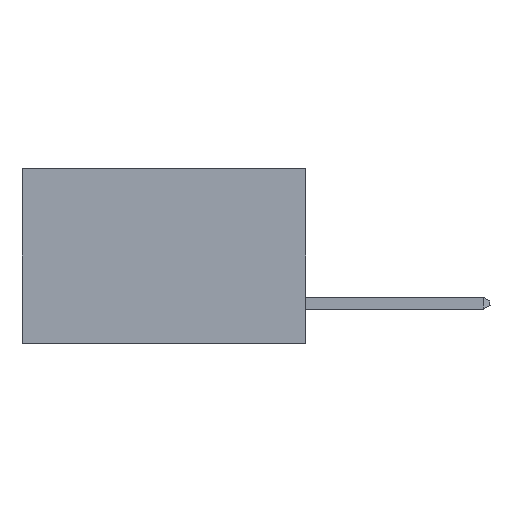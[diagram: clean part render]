
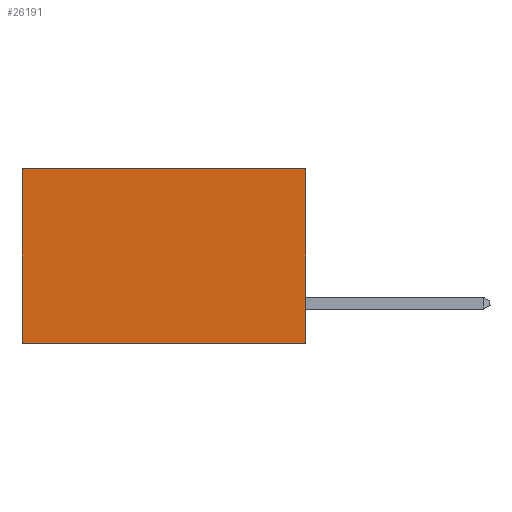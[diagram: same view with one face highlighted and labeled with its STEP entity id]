
A CAD part, left-side view. The second image highlights one B-rep face of the part: STEP entity #26191.
In plain terms, the highlighted planar face has unit normal (-1, 0, 0).
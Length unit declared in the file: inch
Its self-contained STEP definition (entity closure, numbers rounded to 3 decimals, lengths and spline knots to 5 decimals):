
#426 = CARTESIAN_POINT ( 'NONE',  ( 0.298, 0.6, -0.37 ) ) ;
#894 = DIRECTION ( 'NONE',  ( 0., 0., -1. ) ) ;
#2720 = AXIS2_PLACEMENT_3D ( 'NONE', #21661, #5537, #14625 ) ;
#3029 = EDGE_CURVE ( 'NONE', #17017, #24754, #12024, .T. ) ;
#3917 = CARTESIAN_POINT ( 'NONE',  ( 0.298, 0.6, 0. ) ) ;
#4446 = DIRECTION ( 'NONE',  ( 0., 1., 0. ) ) ;
#5003 = CARTESIAN_POINT ( 'NONE',  ( 0.298, 0., 0. ) ) ;
#5537 = DIRECTION ( 'NONE',  ( 1., 0., 0. ) ) ;
#5714 = VECTOR ( 'NONE', #4446, 39.37008 ) ;
#8682 = CARTESIAN_POINT ( 'NONE',  ( 0.298, 0., -0.37 ) ) ;
#9022 = CARTESIAN_POINT ( 'NONE',  ( 0.298, 0., 0. ) ) ;
#11300 = EDGE_LOOP ( 'NONE', ( #22721, #17931, #28256, #11448 ) ) ;
#11448 = ORIENTED_EDGE ( 'NONE', *, *, #27138, .T. ) ;
#11479 = EDGE_CURVE ( 'NONE', #24754, #17449, #12003, .T. ) ;
#12003 = LINE ( 'NONE', #8682, #5714 ) ;
#12024 = LINE ( 'NONE', #21938, #17162 ) ;
#13324 = VECTOR ( 'NONE', #18178, 39.37008 ) ;
#13957 = EDGE_CURVE ( 'NONE', #14714, #17449, #14783, .T. ) ;
#14625 = DIRECTION ( 'NONE',  ( 0., 0., -1. ) ) ;
#14714 = VERTEX_POINT ( 'NONE', #16645 ) ;
#14783 = LINE ( 'NONE', #3917, #13324 ) ;
#15176 = FACE_OUTER_BOUND ( 'NONE', #11300, .T. ) ;
#16645 = CARTESIAN_POINT ( 'NONE',  ( 0.298, 0.6, 0. ) ) ;
#17017 = VERTEX_POINT ( 'NONE', #5003 ) ;
#17162 = VECTOR ( 'NONE', #894, 39.37008 ) ;
#17449 = VERTEX_POINT ( 'NONE', #426 ) ;
#17931 = ORIENTED_EDGE ( 'NONE', *, *, #11479, .F. ) ;
#18178 = DIRECTION ( 'NONE',  ( 0., 0., -1. ) ) ;
#20281 = LINE ( 'NONE', #9022, #27252 ) ;
#21128 = PLANE ( 'NONE',  #2720 ) ;
#21661 = CARTESIAN_POINT ( 'NONE',  ( 0.298, 0., 0. ) ) ;
#21938 = CARTESIAN_POINT ( 'NONE',  ( 0.298, 0., 0. ) ) ;
#22688 = DIRECTION ( 'NONE',  ( 0., 1., 0. ) ) ;
#22721 = ORIENTED_EDGE ( 'NONE', *, *, #13957, .T. ) ;
#24754 = VERTEX_POINT ( 'NONE', #29921 ) ;
#26191 = ADVANCED_FACE ( 'NONE', ( #15176 ), #21128, .F. ) ;
#27138 = EDGE_CURVE ( 'NONE', #17017, #14714, #20281, .T. ) ;
#27252 = VECTOR ( 'NONE', #22688, 39.37008 ) ;
#28256 = ORIENTED_EDGE ( 'NONE', *, *, #3029, .F. ) ;
#29921 = CARTESIAN_POINT ( 'NONE',  ( 0.298, 0., -0.37 ) ) ;
